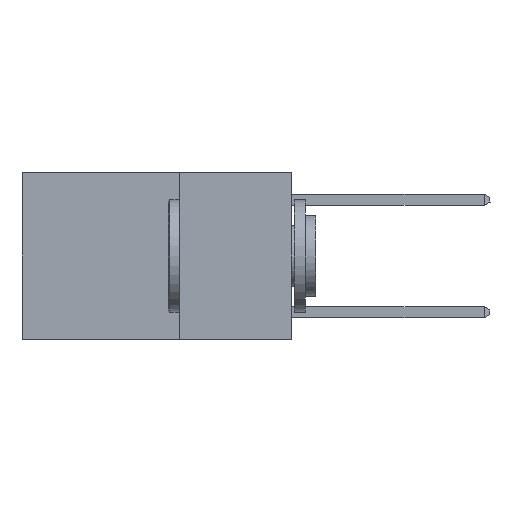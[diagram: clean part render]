
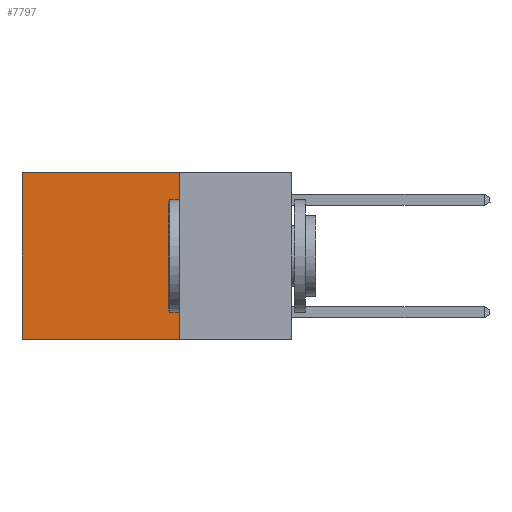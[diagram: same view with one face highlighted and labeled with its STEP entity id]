
A CAD part, left-side view. The second image highlights one B-rep face of the part: STEP entity #7797.
In plain terms, the highlighted planar face has unit normal (-1, 0, 0).
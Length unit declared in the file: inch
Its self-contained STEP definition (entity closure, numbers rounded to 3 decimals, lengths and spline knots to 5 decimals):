
#293 = VERTEX_POINT ( 'NONE', #485 ) ;
#378 = VECTOR ( 'NONE', #14704, 39.37008 ) ;
#485 = CARTESIAN_POINT ( 'NONE',  ( 0.2625, 0.25, -0.37 ) ) ;
#926 = CARTESIAN_POINT ( 'NONE',  ( 0.2625, 0.6, 0. ) ) ;
#1476 = ORIENTED_EDGE ( 'NONE', *, *, #26032, .F. ) ;
#2208 = VECTOR ( 'NONE', #19617, 39.37008 ) ;
#2325 = CARTESIAN_POINT ( 'NONE',  ( 0.2625, 0.25, 0. ) ) ;
#4455 = LINE ( 'NONE', #2325, #2208 ) ;
#4519 = ORIENTED_EDGE ( 'NONE', *, *, #23599, .F. ) ;
#5027 = PLANE ( 'NONE',  #14432 ) ;
#5652 = CARTESIAN_POINT ( 'NONE',  ( 0.2625, 0.6, 0. ) ) ;
#5929 = VERTEX_POINT ( 'NONE', #9230 ) ;
#7797 = ADVANCED_FACE ( 'NONE', ( #19771 ), #5027, .F. ) ;
#8462 = EDGE_CURVE ( 'NONE', #16748, #5929, #23230, .T. ) ;
#9230 = CARTESIAN_POINT ( 'NONE',  ( 0.2625, 0.6, -0.37 ) ) ;
#9383 = EDGE_CURVE ( 'NONE', #13231, #16748, #19323, .T. ) ;
#9546 = DIRECTION ( 'NONE',  ( 0., 0., -1. ) ) ;
#11461 = VECTOR ( 'NONE', #22464, 39.37008 ) ;
#11512 = CARTESIAN_POINT ( 'NONE',  ( 0.2625, 0.25, -0.37 ) ) ;
#13231 = VERTEX_POINT ( 'NONE', #26597 ) ;
#14432 = AXIS2_PLACEMENT_3D ( 'NONE', #22032, #24298, #9546 ) ;
#14704 = DIRECTION ( 'NONE',  ( 0., 0., -1. ) ) ;
#15249 = ORIENTED_EDGE ( 'NONE', *, *, #8462, .T. ) ;
#16492 = EDGE_LOOP ( 'NONE', ( #15249, #4519, #1476, #17721 ) ) ;
#16748 = VERTEX_POINT ( 'NONE', #926 ) ;
#17721 = ORIENTED_EDGE ( 'NONE', *, *, #9383, .T. ) ;
#19323 = LINE ( 'NONE', #27985, #25358 ) ;
#19617 = DIRECTION ( 'NONE',  ( 0., 0., -1. ) ) ;
#19771 = FACE_OUTER_BOUND ( 'NONE', #16492, .T. ) ;
#22032 = CARTESIAN_POINT ( 'NONE',  ( 0.2625, 0.25, 0. ) ) ;
#22464 = DIRECTION ( 'NONE',  ( 0., 1., 0. ) ) ;
#23230 = LINE ( 'NONE', #5652, #378 ) ;
#23599 = EDGE_CURVE ( 'NONE', #293, #5929, #25003, .T. ) ;
#23857 = DIRECTION ( 'NONE',  ( 0., 1., 0. ) ) ;
#24298 = DIRECTION ( 'NONE',  ( 1., 0., 0. ) ) ;
#25003 = LINE ( 'NONE', #11512, #11461 ) ;
#25358 = VECTOR ( 'NONE', #23857, 39.37008 ) ;
#26032 = EDGE_CURVE ( 'NONE', #13231, #293, #4455, .T. ) ;
#26597 = CARTESIAN_POINT ( 'NONE',  ( 0.2625, 0.25, 0. ) ) ;
#27985 = CARTESIAN_POINT ( 'NONE',  ( 0.2625, 0.25, 0. ) ) ;
